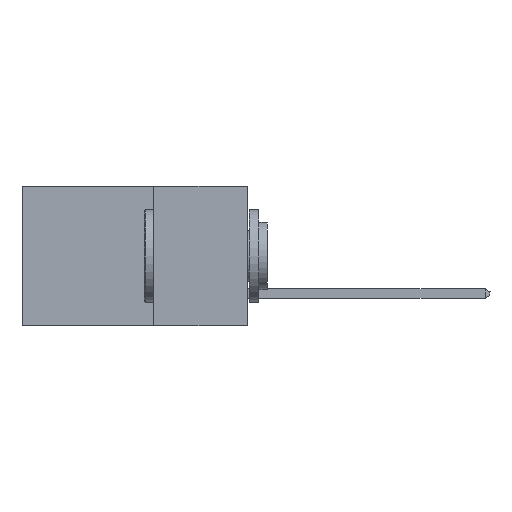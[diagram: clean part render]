
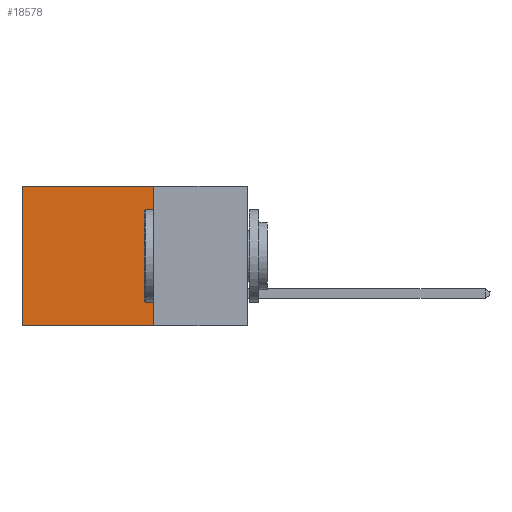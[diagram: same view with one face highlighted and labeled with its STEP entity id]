
A CAD part, left-side view. The second image highlights one B-rep face of the part: STEP entity #18578.
In plain terms, the highlighted planar face has unit normal (-1, 0, 0).
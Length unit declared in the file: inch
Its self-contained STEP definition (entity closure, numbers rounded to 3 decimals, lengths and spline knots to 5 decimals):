
#342 = CARTESIAN_POINT ( 'NONE',  ( 0.2615, 0.25, -0.37 ) ) ;
#1912 = EDGE_CURVE ( 'NONE', #8050, #12341, #8407, .T. ) ;
#1916 = CARTESIAN_POINT ( 'NONE',  ( 0.2615, 0.6, -0.37 ) ) ;
#1984 = AXIS2_PLACEMENT_3D ( 'NONE', #22642, #5043, #4021 ) ;
#3241 = ORIENTED_EDGE ( 'NONE', *, *, #7527, .T. ) ;
#3394 = ORIENTED_EDGE ( 'NONE', *, *, #18965, .T. ) ;
#3678 = DIRECTION ( 'NONE',  ( 0., 1., 0. ) ) ;
#3740 = LINE ( 'NONE', #1916, #4020 ) ;
#4020 = VECTOR ( 'NONE', #9235, 39.37008 ) ;
#4021 = DIRECTION ( 'NONE',  ( 0., 0., -1. ) ) ;
#4204 = DIRECTION ( 'NONE',  ( 0., 0., -1. ) ) ;
#5043 = DIRECTION ( 'NONE',  ( 1., 0., 0. ) ) ;
#5959 = CARTESIAN_POINT ( 'NONE',  ( 0.2615, 0.25, -0.37 ) ) ;
#6627 = EDGE_LOOP ( 'NONE', ( #3241, #8615, #9941, #3394 ) ) ;
#6721 = VERTEX_POINT ( 'NONE', #11776 ) ;
#6971 = FACE_OUTER_BOUND ( 'NONE', #6627, .T. ) ;
#7527 = EDGE_CURVE ( 'NONE', #13667, #6721, #3740, .T. ) ;
#7685 = LINE ( 'NONE', #11655, #13853 ) ;
#8050 = VERTEX_POINT ( 'NONE', #15010 ) ;
#8407 = LINE ( 'NONE', #342, #11748 ) ;
#8615 = ORIENTED_EDGE ( 'NONE', *, *, #21143, .F. ) ;
#9235 = DIRECTION ( 'NONE',  ( 0., 0., -1. ) ) ;
#9353 = DIRECTION ( 'NONE',  ( 0., 1., 0. ) ) ;
#9941 = ORIENTED_EDGE ( 'NONE', *, *, #1912, .F. ) ;
#11385 = CARTESIAN_POINT ( 'NONE',  ( 0.2615, 0.25, -0.37 ) ) ;
#11655 = CARTESIAN_POINT ( 'NONE',  ( 0.2615, 0.25, 0. ) ) ;
#11748 = VECTOR ( 'NONE', #4204, 39.37008 ) ;
#11776 = CARTESIAN_POINT ( 'NONE',  ( 0.2615, 0.6, -0.37 ) ) ;
#12341 = VERTEX_POINT ( 'NONE', #11385 ) ;
#13667 = VERTEX_POINT ( 'NONE', #24443 ) ;
#13853 = VECTOR ( 'NONE', #9353, 39.37008 ) ;
#14761 = VECTOR ( 'NONE', #3678, 39.37008 ) ;
#14816 = PLANE ( 'NONE',  #1984 ) ;
#15010 = CARTESIAN_POINT ( 'NONE',  ( 0.2615, 0.25, 0. ) ) ;
#18578 = ADVANCED_FACE ( 'NONE', ( #6971 ), #14816, .F. ) ;
#18965 = EDGE_CURVE ( 'NONE', #8050, #13667, #7685, .T. ) ;
#19220 = LINE ( 'NONE', #5959, #14761 ) ;
#21143 = EDGE_CURVE ( 'NONE', #12341, #6721, #19220, .T. ) ;
#22642 = CARTESIAN_POINT ( 'NONE',  ( 0.2615, 0.25, -0.37 ) ) ;
#24443 = CARTESIAN_POINT ( 'NONE',  ( 0.2615, 0.6, 0. ) ) ;
